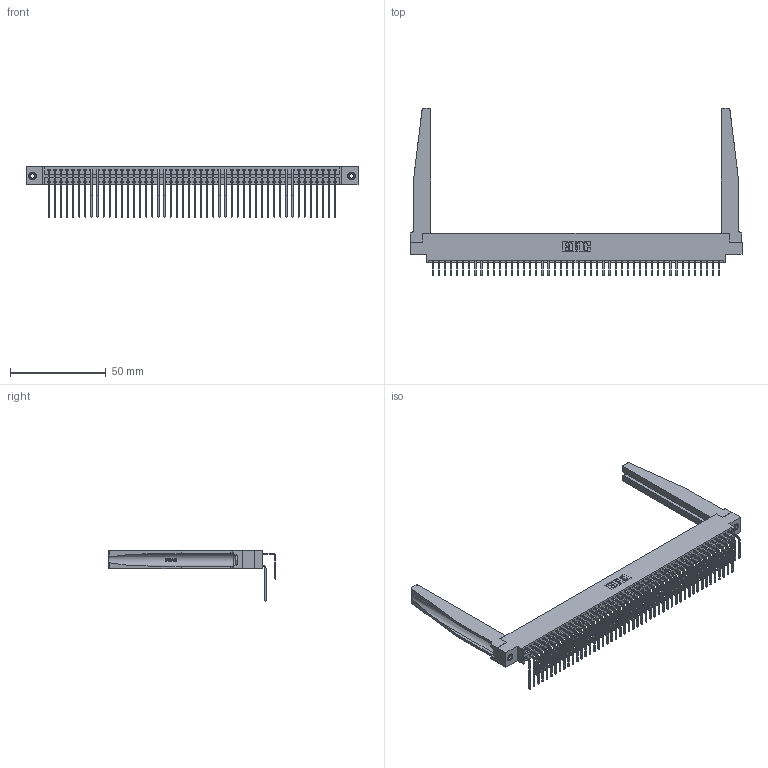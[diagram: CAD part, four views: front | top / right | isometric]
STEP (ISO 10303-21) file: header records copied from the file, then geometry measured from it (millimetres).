
FILE_DESCRIPTION (( 'STEP AP203' ), '1' );
FILE_NAME ('396-096-558-878.STEP', '2019-11-03T15:22:37', ( '' ), ( '' ), 'SwSTEP 2.0', 'SolidWorks 2016', '' );
FILE_SCHEMA (( 'CONFIG_CONTROL_DESIGN' ));
Length unit declared in the file: inch
Products named in the file (6): 345-292-001_558 Tail - 2; 346 Part_0.170 Offset - 0.156 Dia-TH; 345-292-001_558 559 Tail - 1; 396-096-558-878; 346-220-078_345-220-078; 345-250-001_345-250-001-102
Assembly tree (101 placements, depth 2):
  396-096-558-878
    346 Part_0.170 Offset - 0.156 Dia-TH
    345-292-001_558 559 Tail - 1  x48
    345-292-001_558 Tail - 2  x48
    346-220-078_345-220-078  x2
    345-250-001_345-250-001-102  x2
Bounding box: 172.97 x 87.44 x 26.16 mm (x, y, z)
Volume: 24221.8 mm3; surface area: 33266 mm2
Topology: 101 solids, 101 shells, 5544 faces, 16405 edges, 10798 vertices
Faces by surface type: plane 3774, cylinder 1718, bspline 36, cone 12, torus 4
Entity records: 37182 total; most frequent: CARTESIAN_POINT 7110, ORIENTED_EDGE 5882, DIRECTION 5275, EDGE_CURVE 2941, LINE 2483, VECTOR 2483, VERTEX_POINT 1952, AXIS2_PLACEMENT_3D 1396
